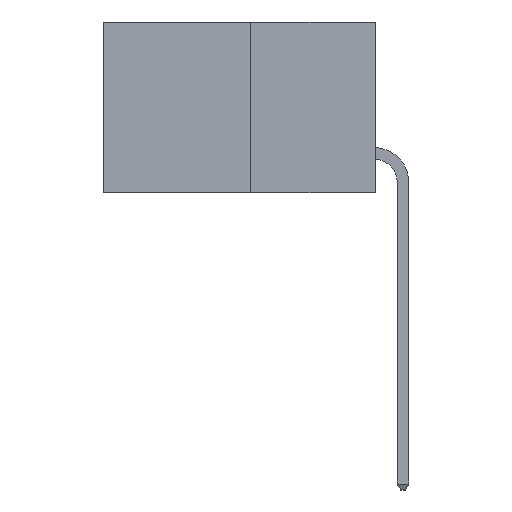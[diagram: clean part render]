
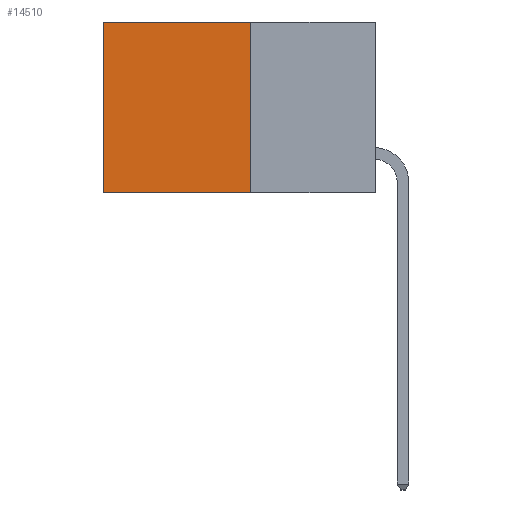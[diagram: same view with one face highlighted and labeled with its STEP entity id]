
A CAD part, left-side view. The second image highlights one B-rep face of the part: STEP entity #14510.
In plain terms, the highlighted planar face has unit normal (-1, 0, 0).
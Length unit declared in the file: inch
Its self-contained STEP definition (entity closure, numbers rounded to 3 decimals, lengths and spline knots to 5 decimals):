
#2502 = FACE_OUTER_BOUND ( 'NONE', #14144, .T. ) ;
#4319 = CARTESIAN_POINT ( 'NONE',  ( 0.277, 0.27, 0. ) ) ;
#4561 = CARTESIAN_POINT ( 'NONE',  ( 0.277, 0.27, 0. ) ) ;
#5608 = DIRECTION ( 'NONE',  ( 0., 1., 0. ) ) ;
#6103 = EDGE_CURVE ( 'NONE', #8176, #18290, #7667, .T. ) ;
#6565 = DIRECTION ( 'NONE',  ( 0., 1., 0. ) ) ;
#7493 = ORIENTED_EDGE ( 'NONE', *, *, #19713, .F. ) ;
#7667 = LINE ( 'NONE', #24788, #17424 ) ;
#7908 = ORIENTED_EDGE ( 'NONE', *, *, #15078, .T. ) ;
#8176 = VERTEX_POINT ( 'NONE', #4319 ) ;
#8577 = PLANE ( 'NONE',  #19809 ) ;
#8780 = CARTESIAN_POINT ( 'NONE',  ( 0.277, 0.27, -0.37 ) ) ;
#9400 = VERTEX_POINT ( 'NONE', #11946 ) ;
#10237 = CARTESIAN_POINT ( 'NONE',  ( 0.277, 0.59, -0.37 ) ) ;
#10528 = DIRECTION ( 'NONE',  ( 1., 0., 0. ) ) ;
#11946 = CARTESIAN_POINT ( 'NONE',  ( 0.277, 0.59, -0.37 ) ) ;
#12395 = VECTOR ( 'NONE', #5608, 39.37008 ) ;
#12537 = VERTEX_POINT ( 'NONE', #18703 ) ;
#12713 = ORIENTED_EDGE ( 'NONE', *, *, #6103, .F. ) ;
#14144 = EDGE_LOOP ( 'NONE', ( #7908, #7493, #12713, #21300 ) ) ;
#14510 = ADVANCED_FACE ( 'NONE', ( #2502 ), #8577, .F. ) ;
#15078 = EDGE_CURVE ( 'NONE', #12537, #9400, #24874, .T. ) ;
#15163 = EDGE_CURVE ( 'NONE', #8176, #12537, #18162, .T. ) ;
#17424 = VECTOR ( 'NONE', #18452, 39.37008 ) ;
#17514 = LINE ( 'NONE', #22864, #12395 ) ;
#17570 = VECTOR ( 'NONE', #6565, 39.37008 ) ;
#17969 = DIRECTION ( 'NONE',  ( 0., 0., -1. ) ) ;
#18162 = LINE ( 'NONE', #4561, #17570 ) ;
#18290 = VERTEX_POINT ( 'NONE', #8780 ) ;
#18452 = DIRECTION ( 'NONE',  ( 0., 0., -1. ) ) ;
#18703 = CARTESIAN_POINT ( 'NONE',  ( 0.277, 0.59, 0. ) ) ;
#19713 = EDGE_CURVE ( 'NONE', #18290, #9400, #17514, .T. ) ;
#19809 = AXIS2_PLACEMENT_3D ( 'NONE', #22025, #10528, #23865 ) ;
#19930 = VECTOR ( 'NONE', #17969, 39.37008 ) ;
#21300 = ORIENTED_EDGE ( 'NONE', *, *, #15163, .T. ) ;
#22025 = CARTESIAN_POINT ( 'NONE',  ( 0.277, 0.27, -0.37 ) ) ;
#22864 = CARTESIAN_POINT ( 'NONE',  ( 0.277, 0.27, -0.37 ) ) ;
#23865 = DIRECTION ( 'NONE',  ( 0., 0., -1. ) ) ;
#24788 = CARTESIAN_POINT ( 'NONE',  ( 0.277, 0.27, -0.37 ) ) ;
#24874 = LINE ( 'NONE', #10237, #19930 ) ;
